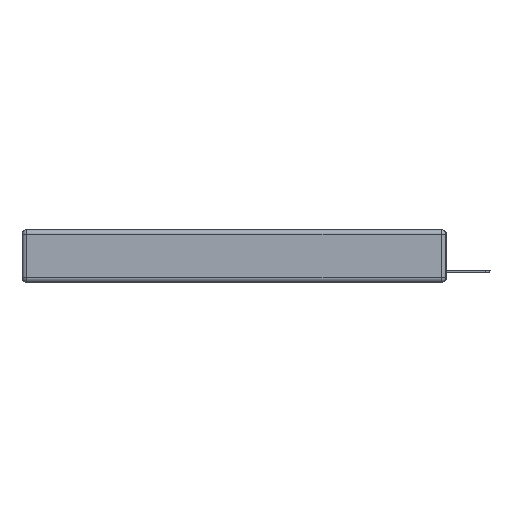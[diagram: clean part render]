
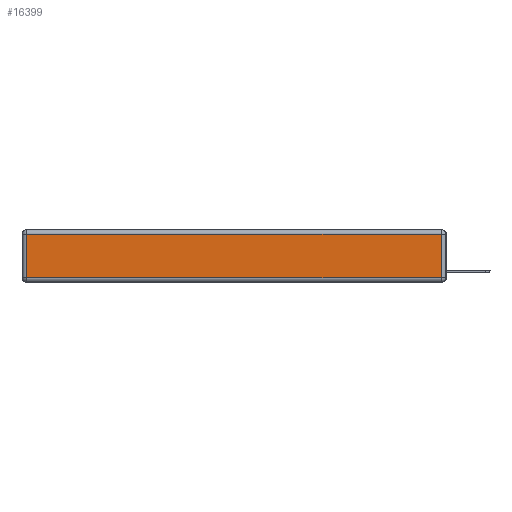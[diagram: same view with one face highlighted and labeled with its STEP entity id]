
A CAD part, left-side view. The second image highlights one B-rep face of the part: STEP entity #16399.
In plain terms, the highlighted planar face has unit normal (-1, 0, 0).
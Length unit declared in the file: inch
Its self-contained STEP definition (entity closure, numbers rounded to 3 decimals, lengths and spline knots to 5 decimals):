
#23 = CARTESIAN_POINT ( 'NONE',  ( 0., 2.72, -0.03 ) ) ;
#685 = VECTOR ( 'NONE', #8567, 39.37008 ) ;
#697 = CARTESIAN_POINT ( 'NONE',  ( 0., 2.75, -0.03 ) ) ;
#719 = DIRECTION ( 'NONE',  ( 0., 0., 1. ) ) ;
#835 = PLANE ( 'NONE',  #16633 ) ;
#931 = LINE ( 'NONE', #697, #685 ) ;
#1326 = CARTESIAN_POINT ( 'NONE',  ( 0., 0.03, -0.313 ) ) ;
#1540 = CARTESIAN_POINT ( 'NONE',  ( 0., 0., -0.313 ) ) ;
#4854 = DIRECTION ( 'NONE',  ( 0., 0., -1. ) ) ;
#5509 = VERTEX_POINT ( 'NONE', #14070 ) ;
#6089 = EDGE_CURVE ( 'NONE', #20482, #23455, #10873, .T. ) ;
#6345 = ORIENTED_EDGE ( 'NONE', *, *, #6089, .T. ) ;
#6584 = CARTESIAN_POINT ( 'NONE',  ( 0., 0., -0.343 ) ) ;
#7422 = LINE ( 'NONE', #1540, #21175 ) ;
#8567 = DIRECTION ( 'NONE',  ( 0., 1., 0. ) ) ;
#10409 = ORIENTED_EDGE ( 'NONE', *, *, #20341, .T. ) ;
#10442 = VECTOR ( 'NONE', #12716, 39.37008 ) ;
#10873 = LINE ( 'NONE', #22047, #18806 ) ;
#11534 = ORIENTED_EDGE ( 'NONE', *, *, #14607, .T. ) ;
#12716 = DIRECTION ( 'NONE',  ( 0., 0., 1. ) ) ;
#14070 = CARTESIAN_POINT ( 'NONE',  ( 0., 0.03, -0.03 ) ) ;
#14607 = EDGE_CURVE ( 'NONE', #21674, #5509, #22362, .T. ) ;
#16399 = ADVANCED_FACE ( 'NONE', ( #21888 ), #835, .T. ) ;
#16633 = AXIS2_PLACEMENT_3D ( 'NONE', #6584, #23910, #719 ) ;
#16886 = ORIENTED_EDGE ( 'NONE', *, *, #17889, .T. ) ;
#17889 = EDGE_CURVE ( 'NONE', #5509, #20482, #931, .T. ) ;
#18806 = VECTOR ( 'NONE', #4854, 39.37008 ) ;
#19741 = EDGE_LOOP ( 'NONE', ( #10409, #11534, #16886, #6345 ) ) ;
#19752 = CARTESIAN_POINT ( 'NONE',  ( 0., 2.72, -0.313 ) ) ;
#19900 = CARTESIAN_POINT ( 'NONE',  ( 0., 0.03, -0.343 ) ) ;
#20341 = EDGE_CURVE ( 'NONE', #23455, #21674, #7422, .T. ) ;
#20482 = VERTEX_POINT ( 'NONE', #23 ) ;
#21175 = VECTOR ( 'NONE', #22968, 39.37008 ) ;
#21674 = VERTEX_POINT ( 'NONE', #1326 ) ;
#21888 = FACE_OUTER_BOUND ( 'NONE', #19741, .T. ) ;
#22047 = CARTESIAN_POINT ( 'NONE',  ( 0., 2.72, -0.343 ) ) ;
#22362 = LINE ( 'NONE', #19900, #10442 ) ;
#22968 = DIRECTION ( 'NONE',  ( 0., -1., 0. ) ) ;
#23455 = VERTEX_POINT ( 'NONE', #19752 ) ;
#23910 = DIRECTION ( 'NONE',  ( -1., 0., 0. ) ) ;
